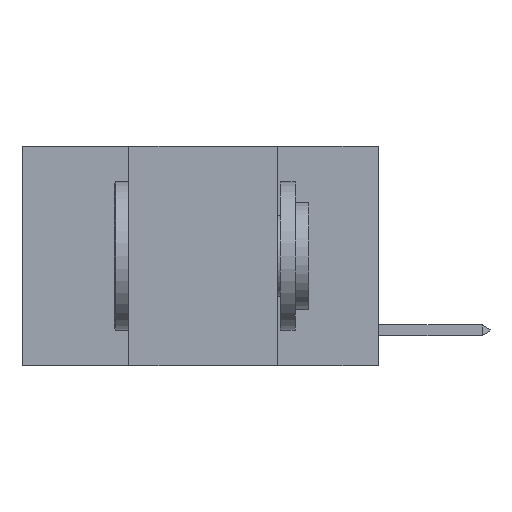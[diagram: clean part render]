
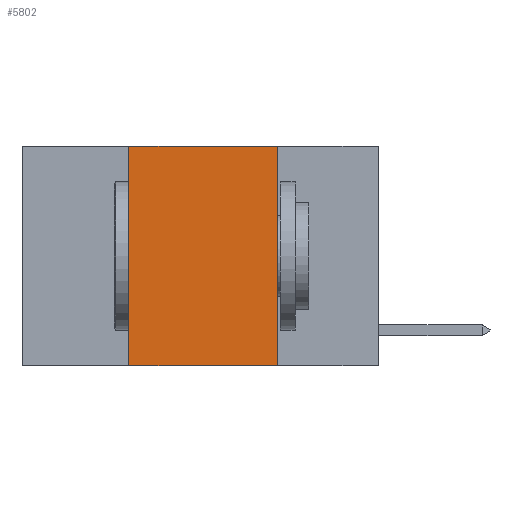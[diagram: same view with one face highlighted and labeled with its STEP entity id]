
A CAD part, left-side view. The second image highlights one B-rep face of the part: STEP entity #5802.
In plain terms, the highlighted planar face has unit normal (-1, 0, 0).
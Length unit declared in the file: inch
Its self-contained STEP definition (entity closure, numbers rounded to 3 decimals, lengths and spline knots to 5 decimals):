
#163 = AXIS2_PLACEMENT_3D ( 'NONE', #8967, #1277, #8053 ) ;
#438 = EDGE_CURVE ( 'NONE', #1751, #2002, #6482, .T. ) ;
#519 = CARTESIAN_POINT ( 'NONE',  ( 0., 0.42, 0. ) ) ;
#857 = CARTESIAN_POINT ( 'NONE',  ( 0., 0.6, 0. ) ) ;
#908 = DIRECTION ( 'NONE',  ( 0., 0., -1. ) ) ;
#918 = CARTESIAN_POINT ( 'NONE',  ( 0., 0.17, 0. ) ) ;
#1277 = DIRECTION ( 'NONE',  ( 1., 0., 0. ) ) ;
#1314 = VECTOR ( 'NONE', #12356, 39.37008 ) ;
#1673 = CARTESIAN_POINT ( 'NONE',  ( 0., 0.17, 0. ) ) ;
#1751 = VERTEX_POINT ( 'NONE', #10448 ) ;
#1820 = ORIENTED_EDGE ( 'NONE', *, *, #438, .F. ) ;
#2002 = VERTEX_POINT ( 'NONE', #519 ) ;
#2084 = LINE ( 'NONE', #6137, #4316 ) ;
#2693 = EDGE_CURVE ( 'NONE', #3178, #8532, #3227, .T. ) ;
#2913 = VECTOR ( 'NONE', #908, 39.37008 ) ;
#3178 = VERTEX_POINT ( 'NONE', #1673 ) ;
#3227 = LINE ( 'NONE', #918, #2913 ) ;
#4187 = CARTESIAN_POINT ( 'NONE',  ( 0., 0.42, 0. ) ) ;
#4316 = VECTOR ( 'NONE', #7116, 39.37008 ) ;
#4360 = ORIENTED_EDGE ( 'NONE', *, *, #5408, .T. ) ;
#4743 = DIRECTION ( 'NONE',  ( 0., -1., 0. ) ) ;
#5187 = EDGE_CURVE ( 'NONE', #2002, #3178, #7413, .T. ) ;
#5408 = EDGE_CURVE ( 'NONE', #1751, #8532, #2084, .T. ) ;
#5802 = ADVANCED_FACE ( 'NONE', ( #9027 ), #10851, .F. ) ;
#6137 = CARTESIAN_POINT ( 'NONE',  ( 0., 0.6, -0.37 ) ) ;
#6482 = LINE ( 'NONE', #4187, #1314 ) ;
#6692 = ORIENTED_EDGE ( 'NONE', *, *, #2693, .F. ) ;
#7116 = DIRECTION ( 'NONE',  ( 0., -1., 0. ) ) ;
#7413 = LINE ( 'NONE', #857, #12107 ) ;
#7898 = EDGE_LOOP ( 'NONE', ( #6692, #9203, #1820, #4360 ) ) ;
#8053 = DIRECTION ( 'NONE',  ( 0., 0., -1. ) ) ;
#8532 = VERTEX_POINT ( 'NONE', #9095 ) ;
#8967 = CARTESIAN_POINT ( 'NONE',  ( 0., 0.6, 0. ) ) ;
#9027 = FACE_OUTER_BOUND ( 'NONE', #7898, .T. ) ;
#9095 = CARTESIAN_POINT ( 'NONE',  ( 0., 0.17, -0.37 ) ) ;
#9203 = ORIENTED_EDGE ( 'NONE', *, *, #5187, .F. ) ;
#10448 = CARTESIAN_POINT ( 'NONE',  ( 0., 0.42, -0.37 ) ) ;
#10851 = PLANE ( 'NONE',  #163 ) ;
#12107 = VECTOR ( 'NONE', #4743, 39.37008 ) ;
#12356 = DIRECTION ( 'NONE',  ( 0., 0., 1. ) ) ;
